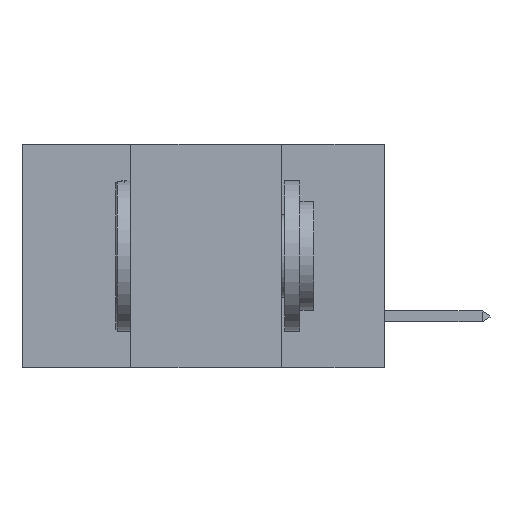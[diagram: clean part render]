
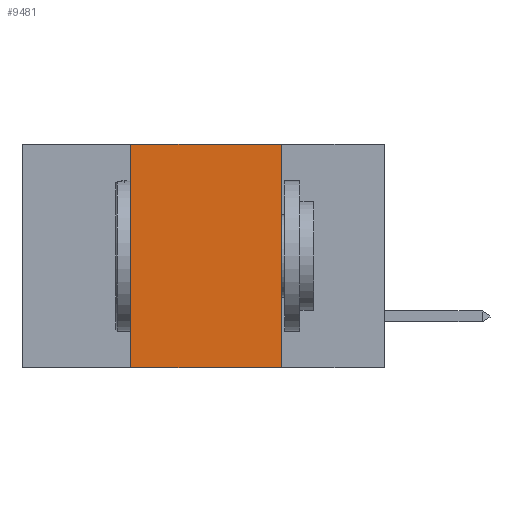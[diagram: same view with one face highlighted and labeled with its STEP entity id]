
A CAD part, left-side view. The second image highlights one B-rep face of the part: STEP entity #9481.
In plain terms, the highlighted planar face has unit normal (-1, 0, 0).
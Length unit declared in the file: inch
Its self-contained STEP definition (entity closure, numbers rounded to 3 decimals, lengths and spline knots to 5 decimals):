
#238 = VECTOR ( 'NONE', #16800, 39.37008 ) ;
#1829 = VECTOR ( 'NONE', #41606, 39.37008 ) ;
#2479 = CARTESIAN_POINT ( 'NONE',  ( 0., 0.6, 0. ) ) ;
#2810 = VECTOR ( 'NONE', #41764, 39.37008 ) ;
#2864 = CARTESIAN_POINT ( 'NONE',  ( 0., 0.17, -0.37 ) ) ;
#5754 = DIRECTION ( 'NONE',  ( 1., 0., 0. ) ) ;
#6345 = VECTOR ( 'NONE', #35578, 39.37008 ) ;
#6437 = VERTEX_POINT ( 'NONE', #38446 ) ;
#9481 = ADVANCED_FACE ( 'NONE', ( #12537 ), #25444, .F. ) ;
#9497 = EDGE_CURVE ( 'NONE', #23302, #17875, #37649, .T. ) ;
#12204 = EDGE_CURVE ( 'NONE', #17875, #31409, #28030, .T. ) ;
#12451 = EDGE_CURVE ( 'NONE', #6437, #23302, #26464, .T. ) ;
#12537 = FACE_OUTER_BOUND ( 'NONE', #30650, .T. ) ;
#13466 = CARTESIAN_POINT ( 'NONE',  ( 0., 0.42, 0. ) ) ;
#14444 = ORIENTED_EDGE ( 'NONE', *, *, #12451, .F. ) ;
#16800 = DIRECTION ( 'NONE',  ( 0., 0., 1. ) ) ;
#17875 = VERTEX_POINT ( 'NONE', #18249 ) ;
#18249 = CARTESIAN_POINT ( 'NONE',  ( 0., 0.17, 0. ) ) ;
#18652 = ORIENTED_EDGE ( 'NONE', *, *, #12204, .F. ) ;
#18824 = CARTESIAN_POINT ( 'NONE',  ( 0., 0.6, 0. ) ) ;
#23302 = VERTEX_POINT ( 'NONE', #36745 ) ;
#23766 = ORIENTED_EDGE ( 'NONE', *, *, #9497, .F. ) ;
#25444 = PLANE ( 'NONE',  #27651 ) ;
#26464 = LINE ( 'NONE', #13466, #238 ) ;
#27651 = AXIS2_PLACEMENT_3D ( 'NONE', #18824, #5754, #28744 ) ;
#28030 = LINE ( 'NONE', #38393, #1829 ) ;
#28744 = DIRECTION ( 'NONE',  ( 0., 0., -1. ) ) ;
#30650 = EDGE_LOOP ( 'NONE', ( #18652, #23766, #14444, #35889 ) ) ;
#30879 = EDGE_CURVE ( 'NONE', #6437, #31409, #32530, .T. ) ;
#31409 = VERTEX_POINT ( 'NONE', #2864 ) ;
#32291 = CARTESIAN_POINT ( 'NONE',  ( 0., 0.6, -0.37 ) ) ;
#32530 = LINE ( 'NONE', #32291, #6345 ) ;
#35578 = DIRECTION ( 'NONE',  ( 0., -1., 0. ) ) ;
#35889 = ORIENTED_EDGE ( 'NONE', *, *, #30879, .T. ) ;
#36745 = CARTESIAN_POINT ( 'NONE',  ( 0., 0.42, 0. ) ) ;
#37649 = LINE ( 'NONE', #2479, #2810 ) ;
#38393 = CARTESIAN_POINT ( 'NONE',  ( 0., 0.17, 0. ) ) ;
#38446 = CARTESIAN_POINT ( 'NONE',  ( 0., 0.42, -0.37 ) ) ;
#41606 = DIRECTION ( 'NONE',  ( 0., 0., -1. ) ) ;
#41764 = DIRECTION ( 'NONE',  ( 0., -1., 0. ) ) ;
